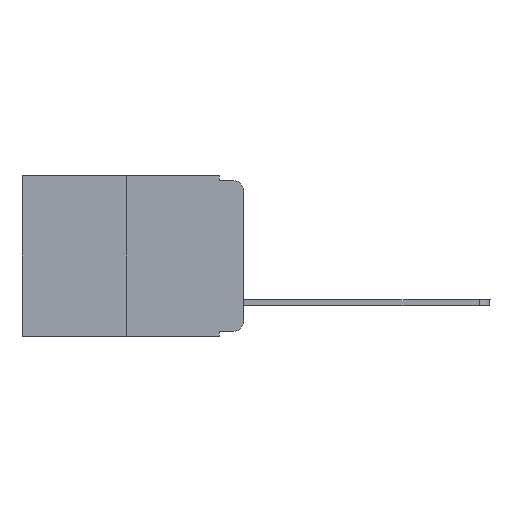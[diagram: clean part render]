
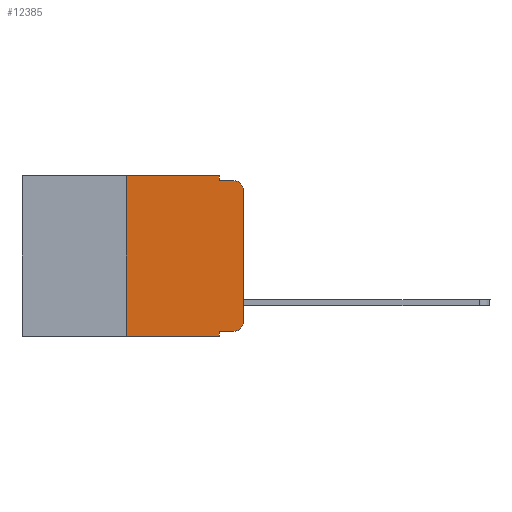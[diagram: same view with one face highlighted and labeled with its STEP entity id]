
A CAD part, left-side view. The second image highlights one B-rep face of the part: STEP entity #12385.
In plain terms, the highlighted planar face has unit normal (-1, 0, 0).
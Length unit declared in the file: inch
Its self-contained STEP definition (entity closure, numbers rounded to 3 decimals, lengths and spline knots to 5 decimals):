
#96 = CARTESIAN_POINT ( 'NONE',  ( 0., 0.051, -0.01 ) ) ;
#186 = ORIENTED_EDGE ( 'NONE', *, *, #7850, .T. ) ;
#231 = DIRECTION ( 'NONE',  ( 0., 0., -1. ) ) ;
#544 = DIRECTION ( 'NONE',  ( 0., 0., 1. ) ) ;
#601 = CARTESIAN_POINT ( 'NONE',  ( 0., 0.473, -0.343 ) ) ;
#784 = CIRCLE ( 'NONE', #12970, 0.02 ) ;
#904 = ORIENTED_EDGE ( 'NONE', *, *, #10459, .T. ) ;
#1041 = DIRECTION ( 'NONE',  ( 1., 0., 0. ) ) ;
#1297 = CARTESIAN_POINT ( 'NONE',  ( 0., 0.051, -0.333 ) ) ;
#1561 = CARTESIAN_POINT ( 'NONE',  ( 0., 0.051, 0. ) ) ;
#1767 = VERTEX_POINT ( 'NONE', #3083 ) ;
#1989 = EDGE_CURVE ( 'NONE', #2274, #9988, #13968, .T. ) ;
#2274 = VERTEX_POINT ( 'NONE', #96 ) ;
#2548 = ORIENTED_EDGE ( 'NONE', *, *, #14621, .F. ) ;
#3001 = AXIS2_PLACEMENT_3D ( 'NONE', #3299, #1041, #5684 ) ;
#3083 = CARTESIAN_POINT ( 'NONE',  ( 0., 0., -0.03 ) ) ;
#3299 = CARTESIAN_POINT ( 'NONE',  ( 0., 0.473, 0. ) ) ;
#3474 = VECTOR ( 'NONE', #544, 39.37008 ) ;
#3518 = VERTEX_POINT ( 'NONE', #12336 ) ;
#3965 = CARTESIAN_POINT ( 'NONE',  ( 0., 0.02, -0.333 ) ) ;
#4016 = DIRECTION ( 'NONE',  ( 0., 0., -1. ) ) ;
#4675 = CARTESIAN_POINT ( 'NONE',  ( 0., 0., 0. ) ) ;
#4861 = LINE ( 'NONE', #9475, #14249 ) ;
#4934 = DIRECTION ( 'NONE',  ( 0., -1., 0. ) ) ;
#5069 = EDGE_LOOP ( 'NONE', ( #186, #7560, #8271, #12344, #2548, #12471, #8583, #7053, #904, #14456 ) ) ;
#5082 = CARTESIAN_POINT ( 'NONE',  ( 0., 0.02, -0.313 ) ) ;
#5297 = DIRECTION ( 'NONE',  ( 0., -1., 0. ) ) ;
#5464 = EDGE_CURVE ( 'NONE', #1767, #9988, #8167, .T. ) ;
#5499 = VERTEX_POINT ( 'NONE', #3965 ) ;
#5684 = DIRECTION ( 'NONE',  ( 0., 0., -1. ) ) ;
#6196 = CARTESIAN_POINT ( 'NONE',  ( 0., 0.051, -0.343 ) ) ;
#6197 = LINE ( 'NONE', #7330, #6665 ) ;
#6539 = VERTEX_POINT ( 'NONE', #8279 ) ;
#6665 = VECTOR ( 'NONE', #11994, 39.37008 ) ;
#7032 = VERTEX_POINT ( 'NONE', #6196 ) ;
#7053 = ORIENTED_EDGE ( 'NONE', *, *, #12135, .F. ) ;
#7330 = CARTESIAN_POINT ( 'NONE',  ( 0., 0.473, 0. ) ) ;
#7352 = LINE ( 'NONE', #1561, #9113 ) ;
#7525 = LINE ( 'NONE', #601, #10049 ) ;
#7560 = ORIENTED_EDGE ( 'NONE', *, *, #5464, .T. ) ;
#7703 = CARTESIAN_POINT ( 'NONE',  ( 0., 0.25, 0. ) ) ;
#7850 = EDGE_CURVE ( 'NONE', #12649, #1767, #10501, .T. ) ;
#8167 = CIRCLE ( 'NONE', #9390, 0.02 ) ;
#8271 = ORIENTED_EDGE ( 'NONE', *, *, #1989, .F. ) ;
#8273 = VECTOR ( 'NONE', #12597, 39.37008 ) ;
#8279 = CARTESIAN_POINT ( 'NONE',  ( 0., 0.051, 0. ) ) ;
#8346 = VECTOR ( 'NONE', #4934, 39.37008 ) ;
#8583 = ORIENTED_EDGE ( 'NONE', *, *, #10612, .T. ) ;
#8783 = LINE ( 'NONE', #7703, #3474 ) ;
#8875 = EDGE_CURVE ( 'NONE', #5499, #12649, #784, .T. ) ;
#9113 = VECTOR ( 'NONE', #11872, 39.37008 ) ;
#9298 = VECTOR ( 'NONE', #14174, 39.37008 ) ;
#9390 = AXIS2_PLACEMENT_3D ( 'NONE', #13088, #9649, #14158 ) ;
#9475 = CARTESIAN_POINT ( 'NONE',  ( 0., 0.051, 0. ) ) ;
#9649 = DIRECTION ( 'NONE',  ( -1., 0., 0. ) ) ;
#9763 = DIRECTION ( 'NONE',  ( -1., 0., 0. ) ) ;
#9988 = VERTEX_POINT ( 'NONE', #14070 ) ;
#10049 = VECTOR ( 'NONE', #5297, 39.37008 ) ;
#10241 = VERTEX_POINT ( 'NONE', #13548 ) ;
#10445 = CARTESIAN_POINT ( 'NONE',  ( 0., 0.051, -0.01 ) ) ;
#10459 = EDGE_CURVE ( 'NONE', #12775, #5499, #11752, .T. ) ;
#10501 = LINE ( 'NONE', #4675, #9298 ) ;
#10612 = EDGE_CURVE ( 'NONE', #10241, #7032, #7525, .T. ) ;
#11100 = CARTESIAN_POINT ( 'NONE',  ( 0., 0.051, -0.333 ) ) ;
#11369 = EDGE_CURVE ( 'NONE', #6539, #2274, #7352, .T. ) ;
#11752 = LINE ( 'NONE', #1297, #8346 ) ;
#11847 = EDGE_CURVE ( 'NONE', #10241, #3518, #8783, .T. ) ;
#11872 = DIRECTION ( 'NONE',  ( 0., 0., -1. ) ) ;
#11994 = DIRECTION ( 'NONE',  ( 0., -1., 0. ) ) ;
#12135 = EDGE_CURVE ( 'NONE', #12775, #7032, #4861, .T. ) ;
#12238 = CARTESIAN_POINT ( 'NONE',  ( 0., 0., -0.313 ) ) ;
#12336 = CARTESIAN_POINT ( 'NONE',  ( 0., 0.25, 0. ) ) ;
#12344 = ORIENTED_EDGE ( 'NONE', *, *, #11369, .F. ) ;
#12385 = ADVANCED_FACE ( 'NONE', ( #12415 ), #13801, .F. ) ;
#12415 = FACE_OUTER_BOUND ( 'NONE', #5069, .T. ) ;
#12471 = ORIENTED_EDGE ( 'NONE', *, *, #11847, .F. ) ;
#12597 = DIRECTION ( 'NONE',  ( 0., -1., 0. ) ) ;
#12649 = VERTEX_POINT ( 'NONE', #12238 ) ;
#12775 = VERTEX_POINT ( 'NONE', #11100 ) ;
#12970 = AXIS2_PLACEMENT_3D ( 'NONE', #5082, #9763, #4016 ) ;
#13088 = CARTESIAN_POINT ( 'NONE',  ( 0., 0.02, -0.03 ) ) ;
#13548 = CARTESIAN_POINT ( 'NONE',  ( 0., 0.25, -0.343 ) ) ;
#13801 = PLANE ( 'NONE',  #3001 ) ;
#13968 = LINE ( 'NONE', #10445, #8273 ) ;
#14070 = CARTESIAN_POINT ( 'NONE',  ( 0., 0.02, -0.01 ) ) ;
#14158 = DIRECTION ( 'NONE',  ( 0., 0., -1. ) ) ;
#14174 = DIRECTION ( 'NONE',  ( 0., 0., 1. ) ) ;
#14249 = VECTOR ( 'NONE', #231, 39.37008 ) ;
#14456 = ORIENTED_EDGE ( 'NONE', *, *, #8875, .T. ) ;
#14621 = EDGE_CURVE ( 'NONE', #3518, #6539, #6197, .T. ) ;
